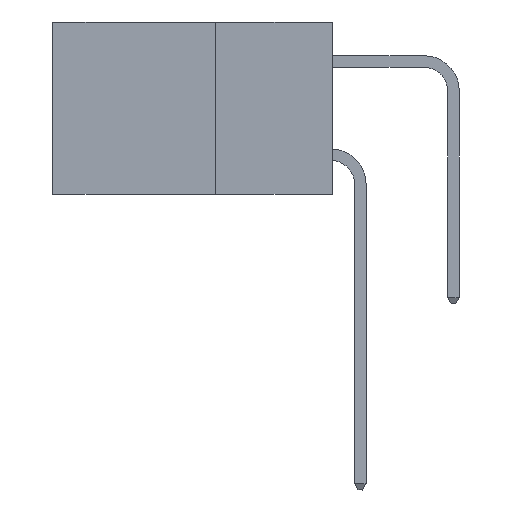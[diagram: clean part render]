
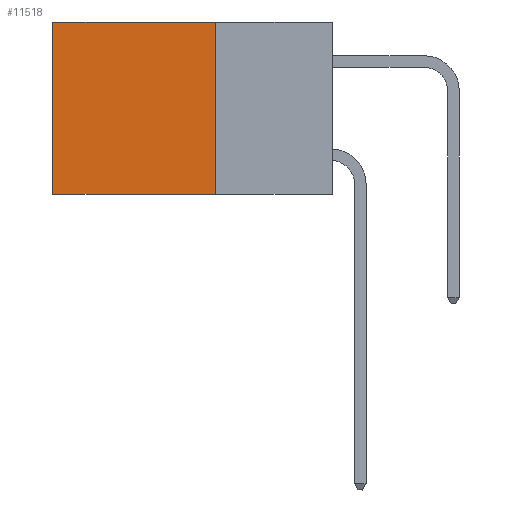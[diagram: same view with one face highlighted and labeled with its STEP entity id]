
A CAD part, left-side view. The second image highlights one B-rep face of the part: STEP entity #11518.
In plain terms, the highlighted planar face has unit normal (-1, 0, 0).
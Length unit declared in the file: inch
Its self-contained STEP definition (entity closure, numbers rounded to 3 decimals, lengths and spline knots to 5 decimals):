
#267 = DIRECTION ( 'NONE',  ( 1., 0., 0. ) ) ;
#1001 = VECTOR ( 'NONE', #16628, 39.37008 ) ;
#1902 = CARTESIAN_POINT ( 'NONE',  ( 0.298, 0.25, 0. ) ) ;
#2682 = CARTESIAN_POINT ( 'NONE',  ( 0.298, 0.6, 0. ) ) ;
#3425 = VECTOR ( 'NONE', #4598, 39.37008 ) ;
#4598 = DIRECTION ( 'NONE',  ( 0., 0., -1. ) ) ;
#4923 = LINE ( 'NONE', #21209, #10551 ) ;
#6599 = FACE_OUTER_BOUND ( 'NONE', #18638, .T. ) ;
#7464 = CARTESIAN_POINT ( 'NONE',  ( 0.298, 0.6, -0.37 ) ) ;
#9091 = ORIENTED_EDGE ( 'NONE', *, *, #18270, .F. ) ;
#9326 = VERTEX_POINT ( 'NONE', #1902 ) ;
#9408 = EDGE_CURVE ( 'NONE', #9326, #14563, #4923, .T. ) ;
#9636 = ORIENTED_EDGE ( 'NONE', *, *, #21717, .T. ) ;
#9760 = PLANE ( 'NONE',  #21779 ) ;
#9859 = DIRECTION ( 'NONE',  ( 0., 0., -1. ) ) ;
#10315 = DIRECTION ( 'NONE',  ( 0., 1., 0. ) ) ;
#10551 = VECTOR ( 'NONE', #9859, 39.37008 ) ;
#11518 = ADVANCED_FACE ( 'NONE', ( #6599 ), #9760, .F. ) ;
#12108 = ORIENTED_EDGE ( 'NONE', *, *, #9408, .F. ) ;
#12908 = VECTOR ( 'NONE', #10315, 39.37008 ) ;
#13506 = LINE ( 'NONE', #2682, #3425 ) ;
#13593 = DIRECTION ( 'NONE',  ( 0., 0., -1. ) ) ;
#14048 = CARTESIAN_POINT ( 'NONE',  ( 0.298, 0.6, 0. ) ) ;
#14563 = VERTEX_POINT ( 'NONE', #23988 ) ;
#16153 = LINE ( 'NONE', #18454, #1001 ) ;
#16628 = DIRECTION ( 'NONE',  ( 0., 1., 0. ) ) ;
#17966 = LINE ( 'NONE', #21576, #12908 ) ;
#18261 = EDGE_CURVE ( 'NONE', #23407, #24285, #13506, .T. ) ;
#18270 = EDGE_CURVE ( 'NONE', #14563, #24285, #17966, .T. ) ;
#18454 = CARTESIAN_POINT ( 'NONE',  ( 0.298, 0.25, 0. ) ) ;
#18638 = EDGE_LOOP ( 'NONE', ( #22417, #9091, #12108, #9636 ) ) ;
#21209 = CARTESIAN_POINT ( 'NONE',  ( 0.298, 0.25, 0. ) ) ;
#21576 = CARTESIAN_POINT ( 'NONE',  ( 0.298, 0.25, -0.37 ) ) ;
#21717 = EDGE_CURVE ( 'NONE', #9326, #23407, #16153, .T. ) ;
#21779 = AXIS2_PLACEMENT_3D ( 'NONE', #23013, #267, #13593 ) ;
#22417 = ORIENTED_EDGE ( 'NONE', *, *, #18261, .T. ) ;
#23013 = CARTESIAN_POINT ( 'NONE',  ( 0.298, 0.25, 0. ) ) ;
#23407 = VERTEX_POINT ( 'NONE', #14048 ) ;
#23988 = CARTESIAN_POINT ( 'NONE',  ( 0.298, 0.25, -0.37 ) ) ;
#24285 = VERTEX_POINT ( 'NONE', #7464 ) ;
